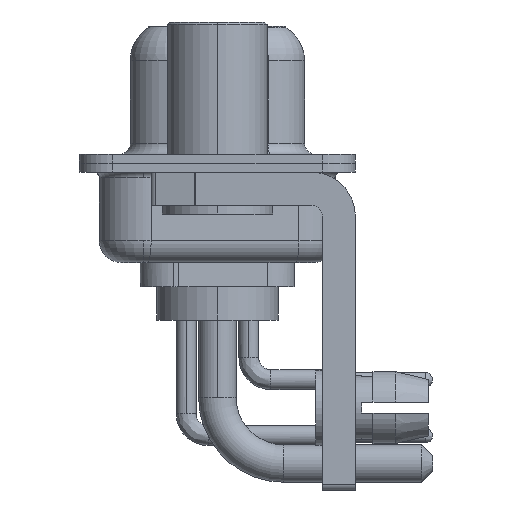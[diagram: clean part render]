
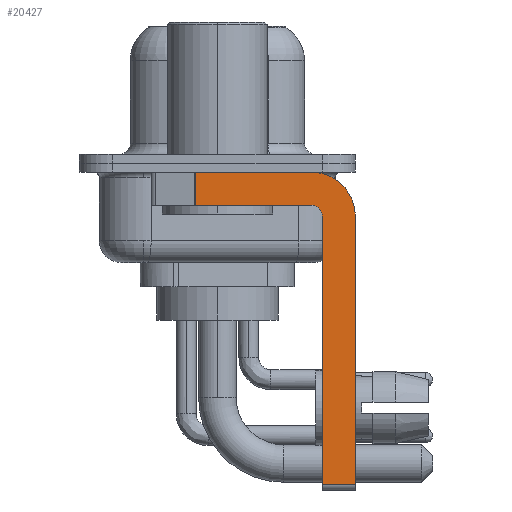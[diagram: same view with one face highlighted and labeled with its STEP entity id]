
A CAD part, left-side view. The second image highlights one B-rep face of the part: STEP entity #20427.
In plain terms, the highlighted planar face has unit normal (-1, 0, 0).
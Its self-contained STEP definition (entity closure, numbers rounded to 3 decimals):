
#29 = VECTOR ( 'NONE', #2134, 1000. ) ;
#55 = DIRECTION ( 'NONE',  ( 1., 0., 0. ) ) ;
#401 = AXIS2_PLACEMENT_3D ( 'NONE', #16943, #563, #17142 ) ;
#510 = EDGE_CURVE ( 'NONE', #14972, #13976, #4715, .T. ) ;
#549 = LINE ( 'NONE', #4014, #7419 ) ;
#563 = DIRECTION ( 'NONE',  ( -1., 0., 0. ) ) ;
#860 = CARTESIAN_POINT ( 'NONE',  ( -2.9, -6.25, -14.55 ) ) ;
#1705 = CARTESIAN_POINT ( 'NONE',  ( -2.9, -4.25, -14.55 ) ) ;
#2134 = DIRECTION ( 'NONE',  ( 0., 0., 1. ) ) ;
#3419 = DIRECTION ( 'NONE',  ( 0., 0., -1. ) ) ;
#3511 = LINE ( 'NONE', #10315, #10176 ) ;
#3618 = DIRECTION ( 'NONE',  ( 0., 0., -1. ) ) ;
#4014 = CARTESIAN_POINT ( 'NONE',  ( -2.9, 3., -0.4 ) ) ;
#4269 = DIRECTION ( 'NONE',  ( 0., 0., -1. ) ) ;
#4315 = VERTEX_POINT ( 'NONE', #4964 ) ;
#4571 = VERTEX_POINT ( 'NONE', #11217 ) ;
#4715 = LINE ( 'NONE', #13156, #9943 ) ;
#4964 = CARTESIAN_POINT ( 'NONE',  ( -2.9, -4.75, -14.55 ) ) ;
#5452 = DIRECTION ( 'NONE',  ( 0., 0., -1. ) ) ;
#6451 = FACE_OUTER_BOUND ( 'NONE', #12921, .T. ) ;
#6681 = EDGE_CURVE ( 'NONE', #7487, #13976, #3511, .T. ) ;
#7419 = VECTOR ( 'NONE', #16038, 1000. ) ;
#7434 = CARTESIAN_POINT ( 'NONE',  ( -2.9, -4.75, -14.8 ) ) ;
#7487 = VERTEX_POINT ( 'NONE', #20020 ) ;
#7837 = VERTEX_POINT ( 'NONE', #19259 ) ;
#7850 = DIRECTION ( 'NONE',  ( 0., 1., 0. ) ) ;
#8106 = LINE ( 'NONE', #1705, #14198 ) ;
#8628 = ORIENTED_EDGE ( 'NONE', *, *, #13326, .T. ) ;
#9743 = ORIENTED_EDGE ( 'NONE', *, *, #16956, .F. ) ;
#9824 = EDGE_CURVE ( 'NONE', #4571, #7837, #12430, .T. ) ;
#9943 = VECTOR ( 'NONE', #7850, 1000. ) ;
#10158 = LINE ( 'NONE', #7434, #29 ) ;
#10161 = DIRECTION ( 'NONE',  ( 0., -1., 0. ) ) ;
#10176 = VECTOR ( 'NONE', #3618, 1000. ) ;
#10215 = CARTESIAN_POINT ( 'NONE',  ( -2.9, -6.25, -2.4 ) ) ;
#10315 = CARTESIAN_POINT ( 'NONE',  ( -2.9, 0.978, -1.9 ) ) ;
#10439 = EDGE_CURVE ( 'NONE', #4315, #13657, #10158, .T. ) ;
#11217 = CARTESIAN_POINT ( 'NONE',  ( -2.9, -4.25, -0.4 ) ) ;
#11542 = CARTESIAN_POINT ( 'NONE',  ( -2.9, -4.25, -1.9 ) ) ;
#11851 = VERTEX_POINT ( 'NONE', #860 ) ;
#11950 = ORIENTED_EDGE ( 'NONE', *, *, #510, .F. ) ;
#12337 = ORIENTED_EDGE ( 'NONE', *, *, #9824, .F. ) ;
#12430 = CIRCLE ( 'NONE', #15189, 2. ) ;
#12921 = EDGE_LOOP ( 'NONE', ( #17323, #16914, #11950, #12974, #13470, #8628, #9743, #12337 ) ) ;
#12974 = ORIENTED_EDGE ( 'NONE', *, *, #14218, .F. ) ;
#13156 = CARTESIAN_POINT ( 'NONE',  ( -2.9, -4.25, -1.9 ) ) ;
#13326 = EDGE_CURVE ( 'NONE', #4315, #11851, #8106, .T. ) ;
#13470 = ORIENTED_EDGE ( 'NONE', *, *, #10439, .F. ) ;
#13657 = VERTEX_POINT ( 'NONE', #14577 ) ;
#13976 = VERTEX_POINT ( 'NONE', #19007 ) ;
#14198 = VECTOR ( 'NONE', #10161, 1000. ) ;
#14218 = EDGE_CURVE ( 'NONE', #13657, #14972, #15264, .T. ) ;
#14577 = CARTESIAN_POINT ( 'NONE',  ( -2.9, -4.75, -2.4 ) ) ;
#14971 = LINE ( 'NONE', #10215, #16769 ) ;
#14972 = VERTEX_POINT ( 'NONE', #11542 ) ;
#15189 = AXIS2_PLACEMENT_3D ( 'NONE', #15856, #20744, #4269 ) ;
#15264 = CIRCLE ( 'NONE', #401, 0.5 ) ;
#15856 = CARTESIAN_POINT ( 'NONE',  ( -2.9, -4.25, -2.4 ) ) ;
#16038 = DIRECTION ( 'NONE',  ( 0., -1., 0. ) ) ;
#16144 = AXIS2_PLACEMENT_3D ( 'NONE', #16628, #55, #3419 ) ;
#16628 = CARTESIAN_POINT ( 'NONE',  ( -2.9, -4.25, -2.4 ) ) ;
#16769 = VECTOR ( 'NONE', #5452, 1000. ) ;
#16914 = ORIENTED_EDGE ( 'NONE', *, *, #6681, .T. ) ;
#16943 = CARTESIAN_POINT ( 'NONE',  ( -2.9, -4.25, -2.4 ) ) ;
#16956 = EDGE_CURVE ( 'NONE', #7837, #11851, #14971, .T. ) ;
#17142 = DIRECTION ( 'NONE',  ( 0., 0., 1. ) ) ;
#17323 = ORIENTED_EDGE ( 'NONE', *, *, #19018, .F. ) ;
#18148 = PLANE ( 'NONE',  #16144 ) ;
#19007 = CARTESIAN_POINT ( 'NONE',  ( -2.9, 0.978, -1.9 ) ) ;
#19018 = EDGE_CURVE ( 'NONE', #7487, #4571, #549, .T. ) ;
#19259 = CARTESIAN_POINT ( 'NONE',  ( -2.9, -6.25, -2.4 ) ) ;
#20020 = CARTESIAN_POINT ( 'NONE',  ( -2.9, 0.978, -0.4 ) ) ;
#20427 = ADVANCED_FACE ( 'NONE', ( #6451 ), #18148, .F. ) ;
#20744 = DIRECTION ( 'NONE',  ( 1., 0., 0. ) ) ;
